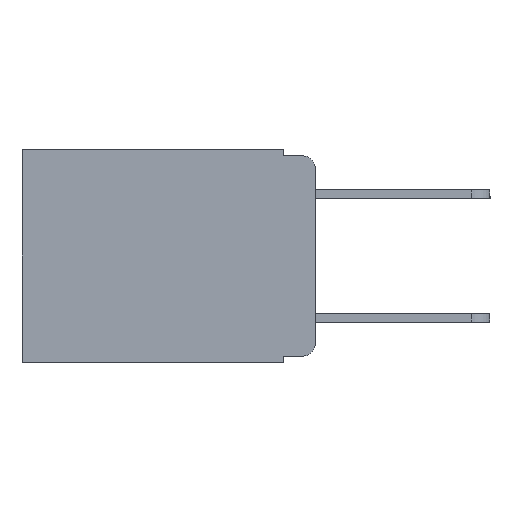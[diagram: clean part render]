
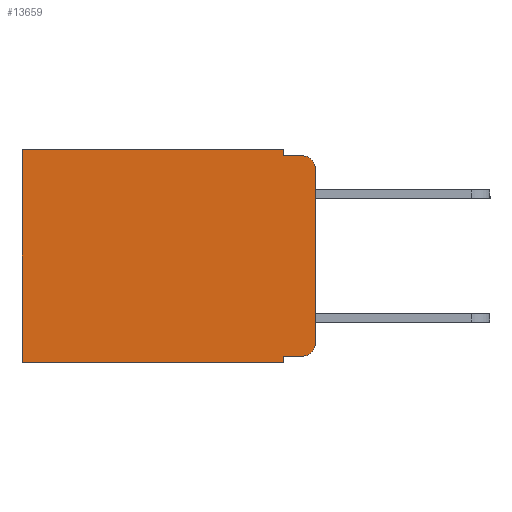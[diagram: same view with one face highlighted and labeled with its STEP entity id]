
A CAD part, left-side view. The second image highlights one B-rep face of the part: STEP entity #13659.
In plain terms, the highlighted planar face has unit normal (-1, 0, 0).
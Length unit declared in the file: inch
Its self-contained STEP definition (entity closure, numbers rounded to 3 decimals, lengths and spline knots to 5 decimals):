
#197 = CARTESIAN_POINT ( 'NONE',  ( 0.298, 0.051, -0.333 ) ) ;
#306 = EDGE_LOOP ( 'NONE', ( #3908, #7421, #7327, #12143, #9560, #5947, #5207, #4330, #1239, #3055 ) ) ;
#322 = DIRECTION ( 'NONE',  ( 0., 0., -1. ) ) ;
#364 = VERTEX_POINT ( 'NONE', #12912 ) ;
#487 = LINE ( 'NONE', #11020, #2889 ) ;
#591 = LINE ( 'NONE', #9891, #8921 ) ;
#708 = DIRECTION ( 'NONE',  ( 0., 0., -1. ) ) ;
#865 = EDGE_CURVE ( 'NONE', #3491, #1734, #4238, .T. ) ;
#1021 = CARTESIAN_POINT ( 'NONE',  ( 0.298, 0.02, -0.313 ) ) ;
#1067 = DIRECTION ( 'NONE',  ( -1., 0., 0. ) ) ;
#1129 = VERTEX_POINT ( 'NONE', #6663 ) ;
#1228 = VERTEX_POINT ( 'NONE', #12203 ) ;
#1239 = ORIENTED_EDGE ( 'NONE', *, *, #6977, .T. ) ;
#1352 = EDGE_CURVE ( 'NONE', #364, #1228, #2028, .T. ) ;
#1501 = VECTOR ( 'NONE', #5404, 39.37008 ) ;
#1734 = VERTEX_POINT ( 'NONE', #8192 ) ;
#1754 = CARTESIAN_POINT ( 'NONE',  ( 0.298, 0.473, 0. ) ) ;
#1790 = DIRECTION ( 'NONE',  ( 0., 0., -1. ) ) ;
#1831 = VERTEX_POINT ( 'NONE', #9846 ) ;
#2028 = CIRCLE ( 'NONE', #3664, 0.02 ) ;
#2646 = CARTESIAN_POINT ( 'NONE',  ( 0.298, 0.473, 0. ) ) ;
#2889 = VECTOR ( 'NONE', #322, 39.37008 ) ;
#3055 = ORIENTED_EDGE ( 'NONE', *, *, #1352, .T. ) ;
#3278 = CARTESIAN_POINT ( 'NONE',  ( 0.298, 0.051, -0.343 ) ) ;
#3491 = VERTEX_POINT ( 'NONE', #13603 ) ;
#3510 = EDGE_CURVE ( 'NONE', #1129, #4313, #9127, .T. ) ;
#3664 = AXIS2_PLACEMENT_3D ( 'NONE', #1021, #1067, #3674 ) ;
#3674 = DIRECTION ( 'NONE',  ( 0., 0., -1. ) ) ;
#3908 = ORIENTED_EDGE ( 'NONE', *, *, #12760, .F. ) ;
#3941 = EDGE_CURVE ( 'NONE', #1129, #12141, #487, .T. ) ;
#4238 = CIRCLE ( 'NONE', #11691, 0.02 ) ;
#4246 = PLANE ( 'NONE',  #9244 ) ;
#4313 = VERTEX_POINT ( 'NONE', #2646 ) ;
#4330 = ORIENTED_EDGE ( 'NONE', *, *, #7637, .F. ) ;
#4993 = EDGE_CURVE ( 'NONE', #12141, #1734, #10421, .T. ) ;
#5173 = LINE ( 'NONE', #197, #7255 ) ;
#5190 = VECTOR ( 'NONE', #12094, 39.37008 ) ;
#5207 = ORIENTED_EDGE ( 'NONE', *, *, #5354, .F. ) ;
#5354 = EDGE_CURVE ( 'NONE', #10591, #5991, #591, .T. ) ;
#5404 = DIRECTION ( 'NONE',  ( 0., 0., -1. ) ) ;
#5947 = ORIENTED_EDGE ( 'NONE', *, *, #6812, .T. ) ;
#5991 = VERTEX_POINT ( 'NONE', #12101 ) ;
#6364 = DIRECTION ( 'NONE',  ( 0., -1., 0. ) ) ;
#6663 = CARTESIAN_POINT ( 'NONE',  ( 0.298, 0.051, 0. ) ) ;
#6752 = VECTOR ( 'NONE', #1790, 39.37008 ) ;
#6812 = EDGE_CURVE ( 'NONE', #4313, #5991, #9325, .T. ) ;
#6856 = VECTOR ( 'NONE', #7061, 39.37008 ) ;
#6977 = EDGE_CURVE ( 'NONE', #1831, #364, #5173, .T. ) ;
#7061 = DIRECTION ( 'NONE',  ( 0., 1., 0. ) ) ;
#7143 = CARTESIAN_POINT ( 'NONE',  ( 0.298, 0., 0. ) ) ;
#7255 = VECTOR ( 'NONE', #6364, 39.37008 ) ;
#7327 = ORIENTED_EDGE ( 'NONE', *, *, #4993, .F. ) ;
#7389 = DIRECTION ( 'NONE',  ( 1., 0., 0. ) ) ;
#7421 = ORIENTED_EDGE ( 'NONE', *, *, #865, .T. ) ;
#7637 = EDGE_CURVE ( 'NONE', #1831, #10591, #7707, .T. ) ;
#7707 = LINE ( 'NONE', #12768, #1501 ) ;
#8192 = CARTESIAN_POINT ( 'NONE',  ( 0.298, 0.02, -0.01 ) ) ;
#8449 = DIRECTION ( 'NONE',  ( 0., 1., 0. ) ) ;
#8921 = VECTOR ( 'NONE', #8449, 39.37008 ) ;
#9046 = FACE_OUTER_BOUND ( 'NONE', #306, .T. ) ;
#9127 = LINE ( 'NONE', #7143, #6856 ) ;
#9244 = AXIS2_PLACEMENT_3D ( 'NONE', #13301, #7389, #708 ) ;
#9325 = LINE ( 'NONE', #1754, #6752 ) ;
#9511 = CARTESIAN_POINT ( 'NONE',  ( 0.298, 0.051, -0.01 ) ) ;
#9560 = ORIENTED_EDGE ( 'NONE', *, *, #3510, .T. ) ;
#9846 = CARTESIAN_POINT ( 'NONE',  ( 0.298, 0.051, -0.333 ) ) ;
#9891 = CARTESIAN_POINT ( 'NONE',  ( 0.298, 0., -0.343 ) ) ;
#10256 = DIRECTION ( 'NONE',  ( 0., 0., -1. ) ) ;
#10421 = LINE ( 'NONE', #10642, #5190 ) ;
#10424 = VECTOR ( 'NONE', #13192, 39.37008 ) ;
#10591 = VERTEX_POINT ( 'NONE', #3278 ) ;
#10642 = CARTESIAN_POINT ( 'NONE',  ( 0.298, 0.051, -0.01 ) ) ;
#10738 = LINE ( 'NONE', #12183, #10424 ) ;
#11020 = CARTESIAN_POINT ( 'NONE',  ( 0.298, 0.051, 0. ) ) ;
#11691 = AXIS2_PLACEMENT_3D ( 'NONE', #12253, #12925, #10256 ) ;
#12094 = DIRECTION ( 'NONE',  ( 0., -1., 0. ) ) ;
#12101 = CARTESIAN_POINT ( 'NONE',  ( 0.298, 0.473, -0.343 ) ) ;
#12141 = VERTEX_POINT ( 'NONE', #9511 ) ;
#12143 = ORIENTED_EDGE ( 'NONE', *, *, #3941, .F. ) ;
#12183 = CARTESIAN_POINT ( 'NONE',  ( 0.298, 0., 0. ) ) ;
#12203 = CARTESIAN_POINT ( 'NONE',  ( 0.298, 0., -0.313 ) ) ;
#12253 = CARTESIAN_POINT ( 'NONE',  ( 0.298, 0.02, -0.03 ) ) ;
#12760 = EDGE_CURVE ( 'NONE', #3491, #1228, #10738, .T. ) ;
#12768 = CARTESIAN_POINT ( 'NONE',  ( 0.298, 0.051, 0. ) ) ;
#12912 = CARTESIAN_POINT ( 'NONE',  ( 0.298, 0.02, -0.333 ) ) ;
#12925 = DIRECTION ( 'NONE',  ( -1., 0., 0. ) ) ;
#13192 = DIRECTION ( 'NONE',  ( 0., 0., -1. ) ) ;
#13301 = CARTESIAN_POINT ( 'NONE',  ( 0.298, 0., 0. ) ) ;
#13603 = CARTESIAN_POINT ( 'NONE',  ( 0.298, 0., -0.03 ) ) ;
#13659 = ADVANCED_FACE ( 'NONE', ( #9046 ), #4246, .F. ) ;
